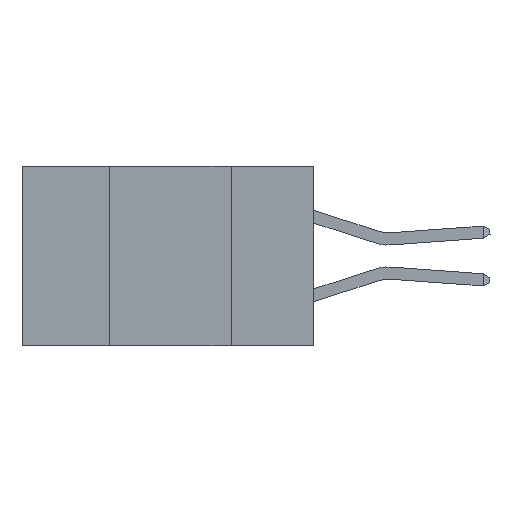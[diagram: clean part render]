
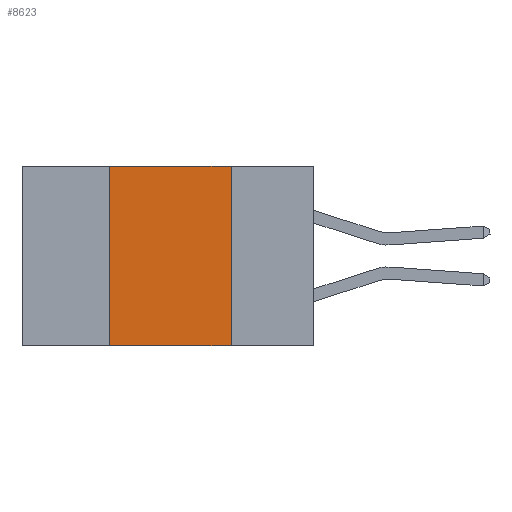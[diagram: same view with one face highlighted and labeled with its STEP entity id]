
A CAD part, left-side view. The second image highlights one B-rep face of the part: STEP entity #8623.
In plain terms, the highlighted planar face has unit normal (-1, 0, 0).
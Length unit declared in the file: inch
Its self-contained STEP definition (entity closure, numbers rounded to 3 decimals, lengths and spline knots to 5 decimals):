
#677 = VERTEX_POINT ( 'NONE', #4968 ) ;
#836 = ORIENTED_EDGE ( 'NONE', *, *, #12969, .F. ) ;
#900 = PLANE ( 'NONE',  #3989 ) ;
#973 = LINE ( 'NONE', #2470, #7726 ) ;
#1274 = VECTOR ( 'NONE', #11290, 39.37008 ) ;
#2125 = LINE ( 'NONE', #6542, #15380 ) ;
#2470 = CARTESIAN_POINT ( 'NONE',  ( 0., 0.6, -0.37 ) ) ;
#3158 = EDGE_CURVE ( 'NONE', #677, #3267, #2125, .T. ) ;
#3267 = VERTEX_POINT ( 'NONE', #10388 ) ;
#3482 = DIRECTION ( 'NONE',  ( 1., 0., 0. ) ) ;
#3555 = EDGE_CURVE ( 'NONE', #10942, #11096, #8600, .T. ) ;
#3771 = DIRECTION ( 'NONE',  ( 0., -1., 0. ) ) ;
#3989 = AXIS2_PLACEMENT_3D ( 'NONE', #11445, #3482, #16711 ) ;
#4968 = CARTESIAN_POINT ( 'NONE',  ( 0., 0.42, -0.37 ) ) ;
#5803 = ORIENTED_EDGE ( 'NONE', *, *, #6491, .T. ) ;
#5978 = LINE ( 'NONE', #8869, #14754 ) ;
#6260 = EDGE_LOOP ( 'NONE', ( #11719, #836, #9269, #5803 ) ) ;
#6491 = EDGE_CURVE ( 'NONE', #677, #11096, #973, .T. ) ;
#6542 = CARTESIAN_POINT ( 'NONE',  ( 0., 0.42, 0. ) ) ;
#6740 = DIRECTION ( 'NONE',  ( 0., -1., 0. ) ) ;
#7726 = VECTOR ( 'NONE', #3771, 39.37008 ) ;
#8531 = CARTESIAN_POINT ( 'NONE',  ( 0., 0.17, 0. ) ) ;
#8600 = LINE ( 'NONE', #16402, #1274 ) ;
#8623 = ADVANCED_FACE ( 'NONE', ( #12855 ), #900, .F. ) ;
#8869 = CARTESIAN_POINT ( 'NONE',  ( 0., 0.6, 0. ) ) ;
#9269 = ORIENTED_EDGE ( 'NONE', *, *, #3158, .F. ) ;
#10388 = CARTESIAN_POINT ( 'NONE',  ( 0., 0.42, 0. ) ) ;
#10942 = VERTEX_POINT ( 'NONE', #8531 ) ;
#11096 = VERTEX_POINT ( 'NONE', #16496 ) ;
#11290 = DIRECTION ( 'NONE',  ( 0., 0., -1. ) ) ;
#11445 = CARTESIAN_POINT ( 'NONE',  ( 0., 0.6, 0. ) ) ;
#11707 = DIRECTION ( 'NONE',  ( 0., 0., 1. ) ) ;
#11719 = ORIENTED_EDGE ( 'NONE', *, *, #3555, .F. ) ;
#12855 = FACE_OUTER_BOUND ( 'NONE', #6260, .T. ) ;
#12969 = EDGE_CURVE ( 'NONE', #3267, #10942, #5978, .T. ) ;
#14754 = VECTOR ( 'NONE', #6740, 39.37008 ) ;
#15380 = VECTOR ( 'NONE', #11707, 39.37008 ) ;
#16402 = CARTESIAN_POINT ( 'NONE',  ( 0., 0.17, 0. ) ) ;
#16496 = CARTESIAN_POINT ( 'NONE',  ( 0., 0.17, -0.37 ) ) ;
#16711 = DIRECTION ( 'NONE',  ( 0., 0., -1. ) ) ;
